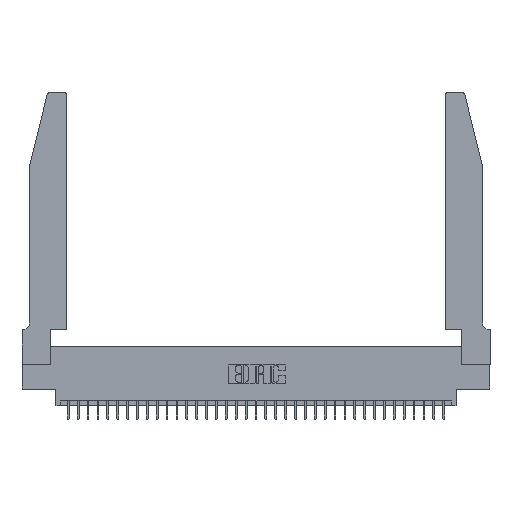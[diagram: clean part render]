
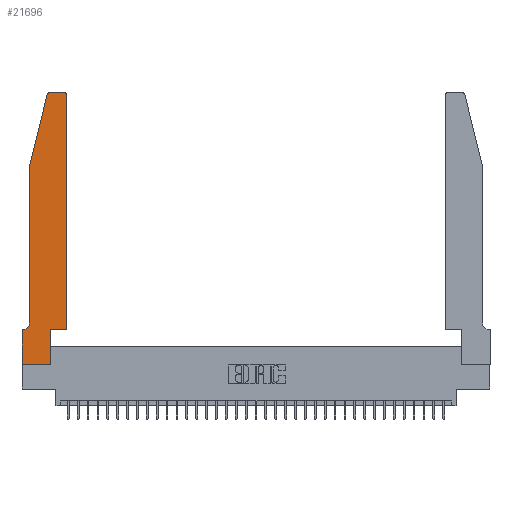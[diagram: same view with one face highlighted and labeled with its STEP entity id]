
A CAD part, top view. The second image highlights one B-rep face of the part: STEP entity #21696.
In plain terms, the highlighted planar face has unit normal (0, 0, 1).
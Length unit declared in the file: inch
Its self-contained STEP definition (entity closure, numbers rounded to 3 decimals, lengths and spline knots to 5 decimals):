
#126 = VECTOR ( 'NONE', #20428, 39.37008 ) ;
#1967 = VERTEX_POINT ( 'NONE', #31281 ) ;
#2043 = EDGE_CURVE ( 'NONE', #1967, #17240, #28050, .T. ) ;
#2908 = VECTOR ( 'NONE', #16585, 39.37008 ) ;
#3263 = DIRECTION ( 'NONE',  ( -1., 0., 0. ) ) ;
#3317 = LINE ( 'NONE', #28442, #21189 ) ;
#3562 = VERTEX_POINT ( 'NONE', #17537 ) ;
#3761 = ORIENTED_EDGE ( 'NONE', *, *, #6149, .T. ) ;
#4845 = VECTOR ( 'NONE', #19636, 39.37008 ) ;
#5016 = DIRECTION ( 'NONE',  ( -1., 0., 0. ) ) ;
#5360 = CARTESIAN_POINT ( 'NONE',  ( 0.0055, 0.42, 0.37 ) ) ;
#5955 = LINE ( 'NONE', #14507, #4845 ) ;
#6069 = VERTEX_POINT ( 'NONE', #19983 ) ;
#6149 = EDGE_CURVE ( 'NONE', #30690, #33032, #5955, .T. ) ;
#6964 = CARTESIAN_POINT ( 'NONE',  ( 0.4505, 0.35, 0.37 ) ) ;
#7039 = CARTESIAN_POINT ( 'NONE',  ( 0.284, 2.75, 0.37 ) ) ;
#7400 = VERTEX_POINT ( 'NONE', #28195 ) ;
#7554 = ORIENTED_EDGE ( 'NONE', *, *, #9931, .T. ) ;
#7871 = ORIENTED_EDGE ( 'NONE', *, *, #32575, .T. ) ;
#7894 = VECTOR ( 'NONE', #14334, 39.37008 ) ;
#7955 = CARTESIAN_POINT ( 'NONE',  ( 0.4205, 2.75, 0.37 ) ) ;
#8059 = ORIENTED_EDGE ( 'NONE', *, *, #32826, .T. ) ;
#8094 = DIRECTION ( 'NONE',  ( -0.239, -0.971, 0. ) ) ;
#8602 = VERTEX_POINT ( 'NONE', #28609 ) ;
#9548 = VECTOR ( 'NONE', #23730, 39.37008 ) ;
#9589 = AXIS2_PLACEMENT_3D ( 'NONE', #34225, #12341, #20899 ) ;
#9931 = EDGE_CURVE ( 'NONE', #33032, #7400, #17729, .T. ) ;
#10566 = VERTEX_POINT ( 'NONE', #30276 ) ;
#10656 = DIRECTION ( 'NONE',  ( 0., 0., -1. ) ) ;
#11232 = VECTOR ( 'NONE', #8094, 39.37008 ) ;
#11637 = VECTOR ( 'NONE', #3263, 39.37008 ) ;
#12341 = DIRECTION ( 'NONE',  ( 0., 0., 1. ) ) ;
#14296 = EDGE_CURVE ( 'NONE', #10566, #6069, #17061, .T. ) ;
#14334 = DIRECTION ( 'NONE',  ( 1., 0., 0. ) ) ;
#14507 = CARTESIAN_POINT ( 'NONE',  ( 0.2605, 2.75, 0.37 ) ) ;
#14762 = CIRCLE ( 'NONE', #35131, 0.07 ) ;
#15341 = CARTESIAN_POINT ( 'NONE',  ( 0., 0., 0.37 ) ) ;
#15914 = LINE ( 'NONE', #27056, #11232 ) ;
#16585 = DIRECTION ( 'NONE',  ( 1., 0., 0. ) ) ;
#16625 = CIRCLE ( 'NONE', #31139, 0.03 ) ;
#16780 = VERTEX_POINT ( 'NONE', #29161 ) ;
#17061 = LINE ( 'NONE', #30361, #7894 ) ;
#17240 = VERTEX_POINT ( 'NONE', #24281 ) ;
#17537 = CARTESIAN_POINT ( 'NONE',  ( 0.0755, 0.42, 0.37 ) ) ;
#17729 = CIRCLE ( 'NONE', #9589, 0.03 ) ;
#17886 = ORIENTED_EDGE ( 'NONE', *, *, #14296, .T. ) ;
#18029 = PLANE ( 'NONE',  #31469 ) ;
#18382 = CARTESIAN_POINT ( 'NONE',  ( 0.4205, 2.72, 0.37 ) ) ;
#18388 = FACE_OUTER_BOUND ( 'NONE', #31340, .T. ) ;
#18450 = LINE ( 'NONE', #15341, #9548 ) ;
#19115 = EDGE_CURVE ( 'NONE', #33479, #16780, #24791, .T. ) ;
#19317 = CARTESIAN_POINT ( 'NONE',  ( 0., 0., 0.37 ) ) ;
#19636 = DIRECTION ( 'NONE',  ( -1., 0., 0. ) ) ;
#19894 = DIRECTION ( 'NONE',  ( 0., -1., 0. ) ) ;
#19983 = CARTESIAN_POINT ( 'NONE',  ( 0.4505, 0.35, 0.37 ) ) ;
#20428 = DIRECTION ( 'NONE',  ( 0., 1., 0. ) ) ;
#20581 = VECTOR ( 'NONE', #34842, 39.37008 ) ;
#20899 = DIRECTION ( 'NONE',  ( 1., 0., 0. ) ) ;
#20917 = DIRECTION ( 'NONE',  ( 1., 0., 0. ) ) ;
#20921 = DIRECTION ( 'NONE',  ( 0., 0., 1. ) ) ;
#21189 = VECTOR ( 'NONE', #19894, 39.37008 ) ;
#21543 = CARTESIAN_POINT ( 'NONE',  ( 0., 0., 0.37 ) ) ;
#21696 = ADVANCED_FACE ( 'NONE', ( #18388 ), #18029, .T. ) ;
#22287 = CARTESIAN_POINT ( 'NONE',  ( 0.0755, 2., 0.37 ) ) ;
#22357 = EDGE_CURVE ( 'NONE', #16780, #10566, #31533, .T. ) ;
#22691 = CARTESIAN_POINT ( 'NONE',  ( 0.2865, 0.35, 0.37 ) ) ;
#22755 = ORIENTED_EDGE ( 'NONE', *, *, #22357, .T. ) ;
#23730 = DIRECTION ( 'NONE',  ( 0., -1., 0. ) ) ;
#24029 = CARTESIAN_POINT ( 'NONE',  ( 0., 0.35, 0.37 ) ) ;
#24281 = CARTESIAN_POINT ( 'NONE',  ( 0., 0.35, 0.37 ) ) ;
#24631 = ORIENTED_EDGE ( 'NONE', *, *, #28163, .T. ) ;
#24791 = LINE ( 'NONE', #19317, #2908 ) ;
#26950 = DIRECTION ( 'NONE',  ( 1., 0., 0. ) ) ;
#27056 = CARTESIAN_POINT ( 'NONE',  ( 0.0755, 2., 0.37 ) ) ;
#27905 = ORIENTED_EDGE ( 'NONE', *, *, #31051, .T. ) ;
#28050 = LINE ( 'NONE', #28217, #11637 ) ;
#28163 = EDGE_CURVE ( 'NONE', #8602, #30690, #16625, .T. ) ;
#28195 = CARTESIAN_POINT ( 'NONE',  ( 0.25487, 2.72718, 0.37 ) ) ;
#28217 = CARTESIAN_POINT ( 'NONE',  ( 0.0755, 0.35, 0.37 ) ) ;
#28442 = CARTESIAN_POINT ( 'NONE',  ( 0.0755, 2., 0.37 ) ) ;
#28609 = CARTESIAN_POINT ( 'NONE',  ( 0.4505, 2.72, 0.37 ) ) ;
#28777 = VERTEX_POINT ( 'NONE', #22287 ) ;
#29161 = CARTESIAN_POINT ( 'NONE',  ( 0.2865, 0., 0.37 ) ) ;
#29665 = DIRECTION ( 'NONE',  ( 0., 0., 1. ) ) ;
#30216 = ORIENTED_EDGE ( 'NONE', *, *, #32319, .T. ) ;
#30223 = ORIENTED_EDGE ( 'NONE', *, *, #2043, .T. ) ;
#30276 = CARTESIAN_POINT ( 'NONE',  ( 0.2865, 0.35, 0.37 ) ) ;
#30361 = CARTESIAN_POINT ( 'NONE',  ( 0.4505, 0.35, 0.37 ) ) ;
#30504 = ORIENTED_EDGE ( 'NONE', *, *, #32579, .T. ) ;
#30690 = VERTEX_POINT ( 'NONE', #7955 ) ;
#31051 = EDGE_CURVE ( 'NONE', #7400, #28777, #15914, .T. ) ;
#31139 = AXIS2_PLACEMENT_3D ( 'NONE', #18382, #29665, #20917 ) ;
#31281 = CARTESIAN_POINT ( 'NONE',  ( 0.0055, 0.35, 0.37 ) ) ;
#31340 = EDGE_LOOP ( 'NONE', ( #3761, #7554, #27905, #8059, #30216, #30223, #30504, #35564, #22755, #17886, #7871, #24631 ) ) ;
#31469 = AXIS2_PLACEMENT_3D ( 'NONE', #24029, #20921, #26950 ) ;
#31533 = LINE ( 'NONE', #22691, #126 ) ;
#31911 = LINE ( 'NONE', #6964, #20581 ) ;
#32319 = EDGE_CURVE ( 'NONE', #3562, #1967, #14762, .T. ) ;
#32575 = EDGE_CURVE ( 'NONE', #6069, #8602, #31911, .T. ) ;
#32579 = EDGE_CURVE ( 'NONE', #17240, #33479, #18450, .T. ) ;
#32826 = EDGE_CURVE ( 'NONE', #28777, #3562, #3317, .T. ) ;
#33032 = VERTEX_POINT ( 'NONE', #7039 ) ;
#33479 = VERTEX_POINT ( 'NONE', #21543 ) ;
#34225 = CARTESIAN_POINT ( 'NONE',  ( 0.284, 2.72, 0.37 ) ) ;
#34842 = DIRECTION ( 'NONE',  ( 0., 1., 0. ) ) ;
#35131 = AXIS2_PLACEMENT_3D ( 'NONE', #5360, #10656, #5016 ) ;
#35564 = ORIENTED_EDGE ( 'NONE', *, *, #19115, .T. ) ;
